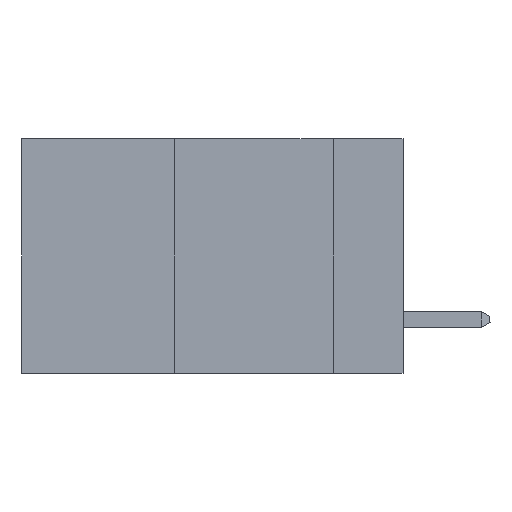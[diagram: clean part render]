
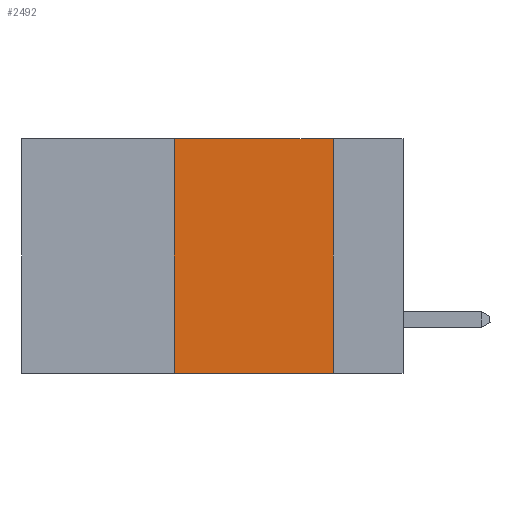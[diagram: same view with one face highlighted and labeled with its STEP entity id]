
A CAD part, left-side view. The second image highlights one B-rep face of the part: STEP entity #2492.
In plain terms, the highlighted planar face has unit normal (-1, 0, 0).
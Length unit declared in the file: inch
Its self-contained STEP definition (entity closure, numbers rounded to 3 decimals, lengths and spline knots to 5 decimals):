
#391 = PLANE ( 'NONE',  #20716 ) ;
#406 = CARTESIAN_POINT ( 'NONE',  ( 0., 0.11, 0. ) ) ;
#544 = VECTOR ( 'NONE', #8617, 39.37008 ) ;
#842 = CARTESIAN_POINT ( 'NONE',  ( 0., 0.6, -0.37 ) ) ;
#1327 = LINE ( 'NONE', #9378, #3132 ) ;
#1860 = LINE ( 'NONE', #10327, #24482 ) ;
#2161 = ORIENTED_EDGE ( 'NONE', *, *, #17150, .F. ) ;
#2346 = CARTESIAN_POINT ( 'NONE',  ( 0., 0.6, 0. ) ) ;
#2492 = ADVANCED_FACE ( 'NONE', ( #6121 ), #391, .F. ) ;
#3132 = VECTOR ( 'NONE', #5375, 39.37008 ) ;
#3656 = CARTESIAN_POINT ( 'NONE',  ( 0., 0.36, -0.37 ) ) ;
#4112 = VECTOR ( 'NONE', #7680, 39.37008 ) ;
#4266 = DIRECTION ( 'NONE',  ( 0., 0., -1. ) ) ;
#4627 = EDGE_CURVE ( 'NONE', #21740, #20832, #1860, .T. ) ;
#5085 = EDGE_CURVE ( 'NONE', #20832, #13865, #7504, .T. ) ;
#5375 = DIRECTION ( 'NONE',  ( 0., 0., -1. ) ) ;
#6094 = EDGE_CURVE ( 'NONE', #21740, #6735, #6593, .T. ) ;
#6121 = FACE_OUTER_BOUND ( 'NONE', #21542, .T. ) ;
#6593 = LINE ( 'NONE', #842, #544 ) ;
#6735 = VERTEX_POINT ( 'NONE', #23623 ) ;
#7504 = LINE ( 'NONE', #9779, #4112 ) ;
#7680 = DIRECTION ( 'NONE',  ( 0., -1., 0. ) ) ;
#8617 = DIRECTION ( 'NONE',  ( 0., -1., 0. ) ) ;
#9274 = ORIENTED_EDGE ( 'NONE', *, *, #6094, .T. ) ;
#9378 = CARTESIAN_POINT ( 'NONE',  ( 0., 0.11, 0. ) ) ;
#9779 = CARTESIAN_POINT ( 'NONE',  ( 0., 0.6, 0. ) ) ;
#10327 = CARTESIAN_POINT ( 'NONE',  ( 0., 0.36, 0. ) ) ;
#11929 = CARTESIAN_POINT ( 'NONE',  ( 0., 0.36, 0. ) ) ;
#12340 = DIRECTION ( 'NONE',  ( 1., 0., 0. ) ) ;
#13865 = VERTEX_POINT ( 'NONE', #406 ) ;
#17150 = EDGE_CURVE ( 'NONE', #13865, #6735, #1327, .T. ) ;
#17906 = DIRECTION ( 'NONE',  ( 0., 0., 1. ) ) ;
#18911 = ORIENTED_EDGE ( 'NONE', *, *, #5085, .F. ) ;
#20716 = AXIS2_PLACEMENT_3D ( 'NONE', #2346, #12340, #4266 ) ;
#20832 = VERTEX_POINT ( 'NONE', #11929 ) ;
#21542 = EDGE_LOOP ( 'NONE', ( #2161, #18911, #24616, #9274 ) ) ;
#21740 = VERTEX_POINT ( 'NONE', #3656 ) ;
#23623 = CARTESIAN_POINT ( 'NONE',  ( 0., 0.11, -0.37 ) ) ;
#24482 = VECTOR ( 'NONE', #17906, 39.37008 ) ;
#24616 = ORIENTED_EDGE ( 'NONE', *, *, #4627, .F. ) ;
